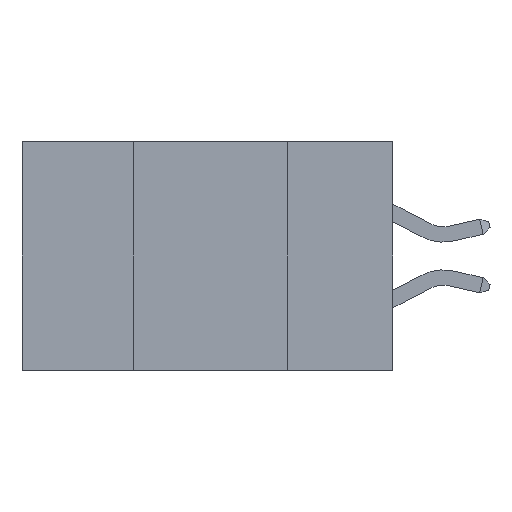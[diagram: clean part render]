
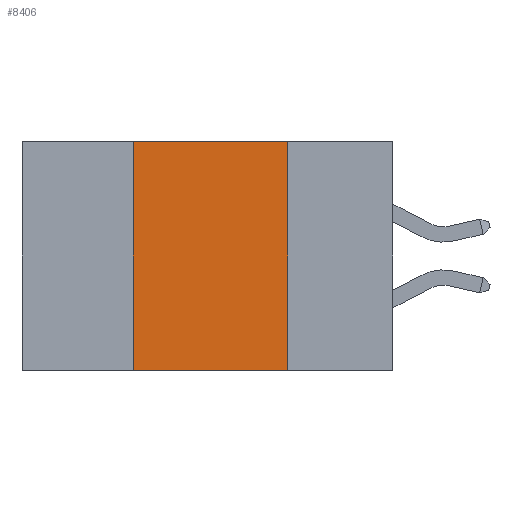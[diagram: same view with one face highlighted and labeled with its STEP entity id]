
A CAD part, left-side view. The second image highlights one B-rep face of the part: STEP entity #8406.
In plain terms, the highlighted planar face has unit normal (-1, 0, 0).
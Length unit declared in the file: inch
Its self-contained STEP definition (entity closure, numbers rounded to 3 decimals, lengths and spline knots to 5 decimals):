
#897 = DIRECTION ( 'NONE',  ( 0., 0., -1. ) ) ;
#1467 = VERTEX_POINT ( 'NONE', #7779 ) ;
#2252 = DIRECTION ( 'NONE',  ( 0., 0., -1. ) ) ;
#2312 = VECTOR ( 'NONE', #6193, 39.37008 ) ;
#3169 = VECTOR ( 'NONE', #15517, 39.37008 ) ;
#3412 = CARTESIAN_POINT ( 'NONE',  ( 0., 0.6, 0. ) ) ;
#3826 = VERTEX_POINT ( 'NONE', #8644 ) ;
#4183 = EDGE_CURVE ( 'NONE', #9621, #1467, #17112, .T. ) ;
#5461 = AXIS2_PLACEMENT_3D ( 'NONE', #15755, #10482, #2252 ) ;
#5861 = EDGE_LOOP ( 'NONE', ( #9290, #9325, #9418, #9432 ) ) ;
#6193 = DIRECTION ( 'NONE',  ( 0., 0., 1. ) ) ;
#6772 = EDGE_CURVE ( 'NONE', #3826, #7576, #11703, .T. ) ;
#7545 = CARTESIAN_POINT ( 'NONE',  ( 0., 0.6, -0.37 ) ) ;
#7576 = VERTEX_POINT ( 'NONE', #9920 ) ;
#7779 = CARTESIAN_POINT ( 'NONE',  ( 0., 0.17, 0. ) ) ;
#8406 = ADVANCED_FACE ( 'NONE', ( #9977 ), #9145, .F. ) ;
#8644 = CARTESIAN_POINT ( 'NONE',  ( 0., 0.42, -0.37 ) ) ;
#9145 = PLANE ( 'NONE',  #5461 ) ;
#9277 = VECTOR ( 'NONE', #14241, 39.37008 ) ;
#9290 = ORIENTED_EDGE ( 'NONE', *, *, #11269, .F. ) ;
#9325 = ORIENTED_EDGE ( 'NONE', *, *, #4183, .F. ) ;
#9418 = ORIENTED_EDGE ( 'NONE', *, *, #13084, .F. ) ;
#9432 = ORIENTED_EDGE ( 'NONE', *, *, #6772, .T. ) ;
#9621 = VERTEX_POINT ( 'NONE', #14198 ) ;
#9920 = CARTESIAN_POINT ( 'NONE',  ( 0., 0.17, -0.37 ) ) ;
#9977 = FACE_OUTER_BOUND ( 'NONE', #5861, .T. ) ;
#10482 = DIRECTION ( 'NONE',  ( 1., 0., 0. ) ) ;
#10595 = CARTESIAN_POINT ( 'NONE',  ( 0., 0.17, 0. ) ) ;
#11269 = EDGE_CURVE ( 'NONE', #1467, #7576, #13710, .T. ) ;
#11703 = LINE ( 'NONE', #7545, #3169 ) ;
#12965 = CARTESIAN_POINT ( 'NONE',  ( 0., 0.42, 0. ) ) ;
#13084 = EDGE_CURVE ( 'NONE', #3826, #9621, #13641, .T. ) ;
#13297 = VECTOR ( 'NONE', #897, 39.37008 ) ;
#13641 = LINE ( 'NONE', #12965, #2312 ) ;
#13710 = LINE ( 'NONE', #10595, #13297 ) ;
#14198 = CARTESIAN_POINT ( 'NONE',  ( 0., 0.42, 0. ) ) ;
#14241 = DIRECTION ( 'NONE',  ( 0., -1., 0. ) ) ;
#15517 = DIRECTION ( 'NONE',  ( 0., -1., 0. ) ) ;
#15755 = CARTESIAN_POINT ( 'NONE',  ( 0., 0.6, 0. ) ) ;
#17112 = LINE ( 'NONE', #3412, #9277 ) ;
